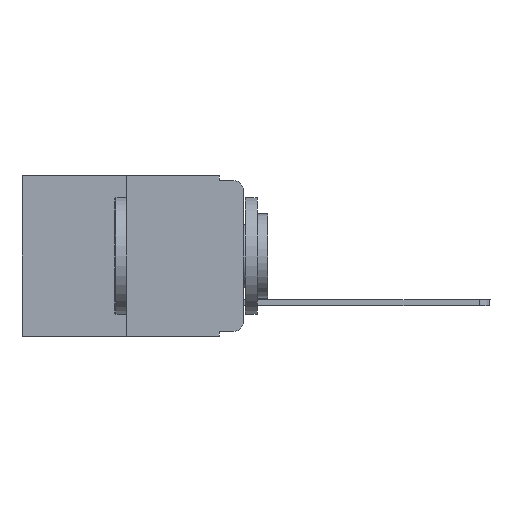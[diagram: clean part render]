
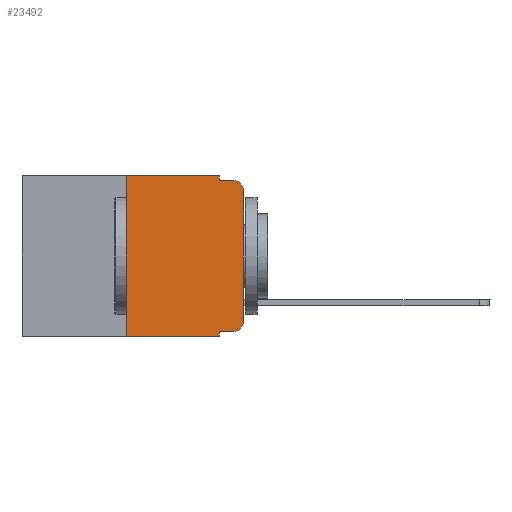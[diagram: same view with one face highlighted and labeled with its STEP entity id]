
A CAD part, left-side view. The second image highlights one B-rep face of the part: STEP entity #23492.
In plain terms, the highlighted planar face has unit normal (-1, 0, 0).
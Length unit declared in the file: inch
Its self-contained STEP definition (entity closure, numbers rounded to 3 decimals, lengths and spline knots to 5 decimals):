
#131 = DIRECTION ( 'NONE',  ( -1., 0., 0. ) ) ;
#441 = VECTOR ( 'NONE', #9651, 39.37008 ) ;
#541 = CARTESIAN_POINT ( 'NONE',  ( 0., 0.051, -0.343 ) ) ;
#1236 = LINE ( 'NONE', #17801, #15266 ) ;
#1384 = DIRECTION ( 'NONE',  ( 0., -1., 0. ) ) ;
#1582 = EDGE_CURVE ( 'NONE', #17217, #20820, #20139, .T. ) ;
#1601 = DIRECTION ( 'NONE',  ( 1., 0., 0. ) ) ;
#1778 = CARTESIAN_POINT ( 'NONE',  ( 0., 0., -0.313 ) ) ;
#2104 = CARTESIAN_POINT ( 'NONE',  ( 0., 0.02, -0.313 ) ) ;
#2202 = VECTOR ( 'NONE', #17379, 39.37008 ) ;
#3371 = VECTOR ( 'NONE', #1384, 39.37008 ) ;
#3544 = EDGE_LOOP ( 'NONE', ( #14092, #11349, #22064, #23335, #22345, #8895, #22941, #15561, #18821, #13934 ) ) ;
#4322 = DIRECTION ( 'NONE',  ( 0., 0., -1. ) ) ;
#4421 = DIRECTION ( 'NONE',  ( 0., -1., 0. ) ) ;
#4554 = VERTEX_POINT ( 'NONE', #9328 ) ;
#4634 = VERTEX_POINT ( 'NONE', #8246 ) ;
#4645 = AXIS2_PLACEMENT_3D ( 'NONE', #9434, #1601, #21456 ) ;
#6178 = VERTEX_POINT ( 'NONE', #12546 ) ;
#7014 = CARTESIAN_POINT ( 'NONE',  ( 0., 0.051, -0.333 ) ) ;
#7056 = VERTEX_POINT ( 'NONE', #8762 ) ;
#7394 = CARTESIAN_POINT ( 'NONE',  ( 0., 0.051, 0. ) ) ;
#7627 = VECTOR ( 'NONE', #14105, 39.37008 ) ;
#7822 = PLANE ( 'NONE',  #4645 ) ;
#7956 = VECTOR ( 'NONE', #24632, 39.37008 ) ;
#7983 = CARTESIAN_POINT ( 'NONE',  ( 0., 0.02, -0.333 ) ) ;
#8246 = CARTESIAN_POINT ( 'NONE',  ( 0., 0.051, 0. ) ) ;
#8387 = CARTESIAN_POINT ( 'NONE',  ( 0., 0.02, -0.03 ) ) ;
#8762 = CARTESIAN_POINT ( 'NONE',  ( 0., 0.051, -0.01 ) ) ;
#8834 = VERTEX_POINT ( 'NONE', #13749 ) ;
#8895 = ORIENTED_EDGE ( 'NONE', *, *, #23011, .F. ) ;
#9028 = EDGE_CURVE ( 'NONE', #12946, #4554, #13245, .T. ) ;
#9288 = CARTESIAN_POINT ( 'NONE',  ( 0., 0.051, 0. ) ) ;
#9328 = CARTESIAN_POINT ( 'NONE',  ( 0., 0., -0.03 ) ) ;
#9434 = CARTESIAN_POINT ( 'NONE',  ( 0., 0.473, 0. ) ) ;
#9651 = DIRECTION ( 'NONE',  ( 0., 0., 1. ) ) ;
#9763 = LINE ( 'NONE', #7394, #11874 ) ;
#10140 = DIRECTION ( 'NONE',  ( 0., -1., 0. ) ) ;
#10306 = EDGE_CURVE ( 'NONE', #7056, #15906, #16515, .T. ) ;
#11255 = FACE_OUTER_BOUND ( 'NONE', #3544, .T. ) ;
#11337 = AXIS2_PLACEMENT_3D ( 'NONE', #2104, #131, #23676 ) ;
#11349 = ORIENTED_EDGE ( 'NONE', *, *, #15824, .T. ) ;
#11771 = DIRECTION ( 'NONE',  ( 0., 0., -1. ) ) ;
#11874 = VECTOR ( 'NONE', #11771, 39.37008 ) ;
#11878 = LINE ( 'NONE', #12578, #7956 ) ;
#12082 = EDGE_CURVE ( 'NONE', #20820, #12946, #15560, .T. ) ;
#12187 = AXIS2_PLACEMENT_3D ( 'NONE', #8387, #14002, #4322 ) ;
#12546 = CARTESIAN_POINT ( 'NONE',  ( 0., 0.25, 0. ) ) ;
#12556 = VECTOR ( 'NONE', #4421, 39.37008 ) ;
#12578 = CARTESIAN_POINT ( 'NONE',  ( 0., 0.25, 0. ) ) ;
#12946 = VERTEX_POINT ( 'NONE', #1778 ) ;
#13245 = LINE ( 'NONE', #25102, #441 ) ;
#13721 = CARTESIAN_POINT ( 'NONE',  ( 0., 0.051, -0.01 ) ) ;
#13749 = CARTESIAN_POINT ( 'NONE',  ( 0., 0.25, -0.343 ) ) ;
#13934 = ORIENTED_EDGE ( 'NONE', *, *, #12082, .T. ) ;
#14002 = DIRECTION ( 'NONE',  ( -1., 0., 0. ) ) ;
#14092 = ORIENTED_EDGE ( 'NONE', *, *, #9028, .T. ) ;
#14105 = DIRECTION ( 'NONE',  ( 0., 0., -1. ) ) ;
#15266 = VECTOR ( 'NONE', #10140, 39.37008 ) ;
#15560 = CIRCLE ( 'NONE', #11337, 0.02 ) ;
#15561 = ORIENTED_EDGE ( 'NONE', *, *, #24924, .F. ) ;
#15824 = EDGE_CURVE ( 'NONE', #4554, #15906, #20135, .T. ) ;
#15906 = VERTEX_POINT ( 'NONE', #20484 ) ;
#15934 = LINE ( 'NONE', #23914, #12556 ) ;
#16515 = LINE ( 'NONE', #13721, #2202 ) ;
#17053 = VERTEX_POINT ( 'NONE', #541 ) ;
#17217 = VERTEX_POINT ( 'NONE', #22786 ) ;
#17379 = DIRECTION ( 'NONE',  ( 0., -1., 0. ) ) ;
#17801 = CARTESIAN_POINT ( 'NONE',  ( 0., 0.473, -0.343 ) ) ;
#18821 = ORIENTED_EDGE ( 'NONE', *, *, #1582, .T. ) ;
#20135 = CIRCLE ( 'NONE', #12187, 0.02 ) ;
#20139 = LINE ( 'NONE', #7014, #3371 ) ;
#20484 = CARTESIAN_POINT ( 'NONE',  ( 0., 0.02, -0.01 ) ) ;
#20820 = VERTEX_POINT ( 'NONE', #7983 ) ;
#21456 = DIRECTION ( 'NONE',  ( 0., 0., -1. ) ) ;
#21740 = EDGE_CURVE ( 'NONE', #6178, #4634, #15934, .T. ) ;
#22064 = ORIENTED_EDGE ( 'NONE', *, *, #10306, .F. ) ;
#22345 = ORIENTED_EDGE ( 'NONE', *, *, #21740, .F. ) ;
#22786 = CARTESIAN_POINT ( 'NONE',  ( 0., 0.051, -0.333 ) ) ;
#22850 = EDGE_CURVE ( 'NONE', #8834, #17053, #1236, .T. ) ;
#22941 = ORIENTED_EDGE ( 'NONE', *, *, #22850, .T. ) ;
#23011 = EDGE_CURVE ( 'NONE', #8834, #6178, #11878, .T. ) ;
#23184 = LINE ( 'NONE', #9288, #7627 ) ;
#23335 = ORIENTED_EDGE ( 'NONE', *, *, #24547, .F. ) ;
#23492 = ADVANCED_FACE ( 'NONE', ( #11255 ), #7822, .F. ) ;
#23676 = DIRECTION ( 'NONE',  ( 0., 0., -1. ) ) ;
#23914 = CARTESIAN_POINT ( 'NONE',  ( 0., 0.473, 0. ) ) ;
#24547 = EDGE_CURVE ( 'NONE', #4634, #7056, #9763, .T. ) ;
#24632 = DIRECTION ( 'NONE',  ( 0., 0., 1. ) ) ;
#24924 = EDGE_CURVE ( 'NONE', #17217, #17053, #23184, .T. ) ;
#25102 = CARTESIAN_POINT ( 'NONE',  ( 0., 0., 0. ) ) ;
